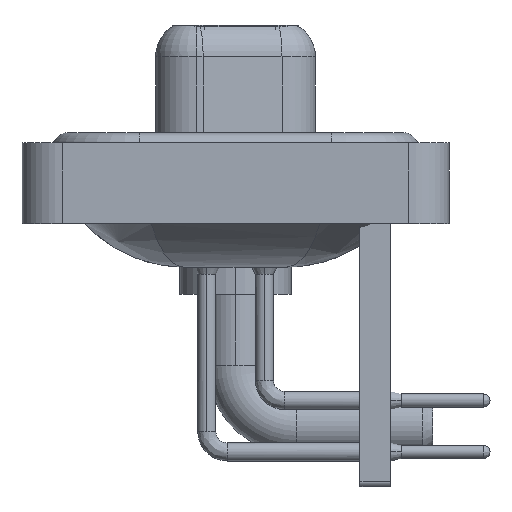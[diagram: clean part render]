
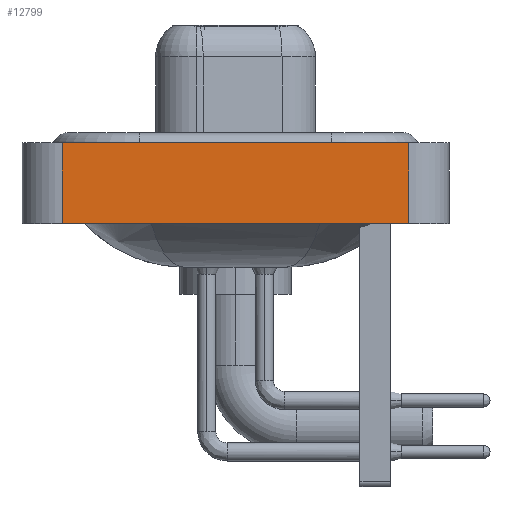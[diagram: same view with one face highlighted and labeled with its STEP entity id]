
A CAD part, left-side view. The second image highlights one B-rep face of the part: STEP entity #12799.
In plain terms, the highlighted planar face has unit normal (-1, 0, 0).
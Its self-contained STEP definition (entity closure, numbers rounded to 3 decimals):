
#119 = LINE ( 'NONE', #21572, #21825 ) ;
#439 = CARTESIAN_POINT ( 'NONE',  ( -7.3, -8.55, 0.4 ) ) ;
#866 = EDGE_CURVE ( 'NONE', #21500, #3592, #8818, .T. ) ;
#1302 = EDGE_CURVE ( 'NONE', #3592, #8592, #119, .T. ) ;
#1998 = DIRECTION ( 'NONE',  ( 0., 0., 1. ) ) ;
#2568 = EDGE_LOOP ( 'NONE', ( #19826, #13389, #9981, #10792 ) ) ;
#2632 = LINE ( 'NONE', #17399, #15682 ) ;
#3296 = CARTESIAN_POINT ( 'NONE',  ( -7.3, 8.55, -3.6 ) ) ;
#3592 = VERTEX_POINT ( 'NONE', #6513 ) ;
#4061 = DIRECTION ( 'NONE',  ( -1., 0., 0. ) ) ;
#4978 = CARTESIAN_POINT ( 'NONE',  ( -7.3, -8.55, -3.6 ) ) ;
#5163 = DIRECTION ( 'NONE',  ( 0., 0., 1. ) ) ;
#5474 = DIRECTION ( 'NONE',  ( 0., 0., 1. ) ) ;
#5809 = CARTESIAN_POINT ( 'NONE',  ( -7.3, -8.55, -3.6 ) ) ;
#6513 = CARTESIAN_POINT ( 'NONE',  ( -7.3, 8.55, 0.4 ) ) ;
#6943 = EDGE_CURVE ( 'NONE', #21500, #11964, #2632, .T. ) ;
#8592 = VERTEX_POINT ( 'NONE', #439 ) ;
#8818 = LINE ( 'NONE', #22738, #20300 ) ;
#9425 = EDGE_CURVE ( 'NONE', #11964, #8592, #19919, .T. ) ;
#9981 = ORIENTED_EDGE ( 'NONE', *, *, #866, .F. ) ;
#10792 = ORIENTED_EDGE ( 'NONE', *, *, #6943, .T. ) ;
#10931 = DIRECTION ( 'NONE',  ( 0., -1., 0. ) ) ;
#11885 = AXIS2_PLACEMENT_3D ( 'NONE', #5809, #4061, #5474 ) ;
#11964 = VERTEX_POINT ( 'NONE', #4978 ) ;
#12799 = ADVANCED_FACE ( 'NONE', ( #12878 ), #19642, .T. ) ;
#12878 = FACE_OUTER_BOUND ( 'NONE', #2568, .T. ) ;
#13389 = ORIENTED_EDGE ( 'NONE', *, *, #1302, .F. ) ;
#13550 = DIRECTION ( 'NONE',  ( 0., -1., 0. ) ) ;
#13712 = VECTOR ( 'NONE', #1998, 1000. ) ;
#15682 = VECTOR ( 'NONE', #13550, 1000. ) ;
#17399 = CARTESIAN_POINT ( 'NONE',  ( -7.3, -8.55, -3.6 ) ) ;
#19468 = CARTESIAN_POINT ( 'NONE',  ( -7.3, -8.55, -3.6 ) ) ;
#19642 = PLANE ( 'NONE',  #11885 ) ;
#19826 = ORIENTED_EDGE ( 'NONE', *, *, #9425, .T. ) ;
#19919 = LINE ( 'NONE', #19468, #13712 ) ;
#20300 = VECTOR ( 'NONE', #5163, 1000. ) ;
#21500 = VERTEX_POINT ( 'NONE', #3296 ) ;
#21572 = CARTESIAN_POINT ( 'NONE',  ( -7.3, -8.55, 0.4 ) ) ;
#21825 = VECTOR ( 'NONE', #10931, 1000. ) ;
#22738 = CARTESIAN_POINT ( 'NONE',  ( -7.3, 8.55, -3.6 ) ) ;
